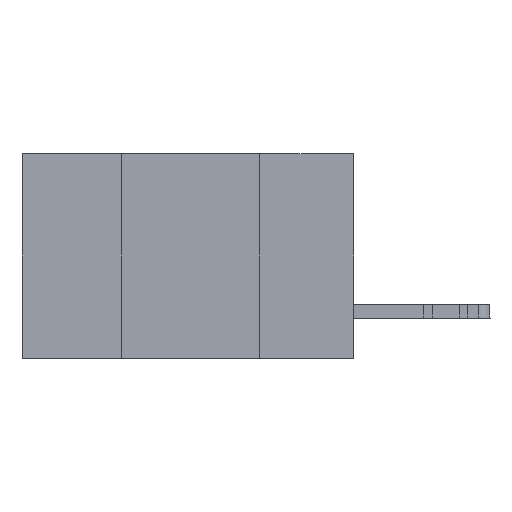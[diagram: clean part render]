
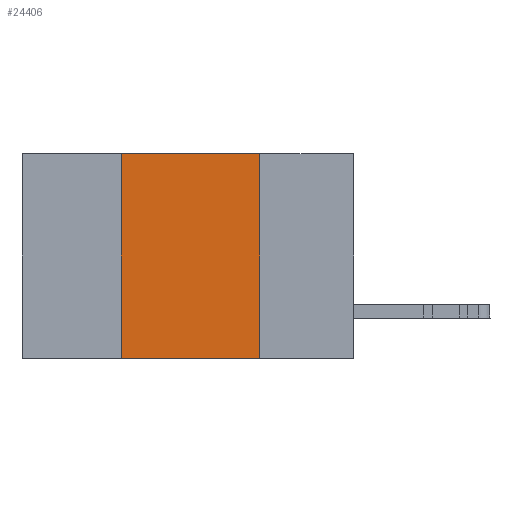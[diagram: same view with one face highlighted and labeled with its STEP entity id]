
A CAD part, left-side view. The second image highlights one B-rep face of the part: STEP entity #24406.
In plain terms, the highlighted planar face has unit normal (-1, 0, 0).
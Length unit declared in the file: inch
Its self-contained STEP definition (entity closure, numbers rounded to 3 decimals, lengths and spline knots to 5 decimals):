
#717 = LINE ( 'NONE', #21312, #35866 ) ;
#966 = EDGE_CURVE ( 'NONE', #1435, #25474, #34516, .T. ) ;
#1435 = VERTEX_POINT ( 'NONE', #48701 ) ;
#3233 = CARTESIAN_POINT ( 'NONE',  ( 0., 0.42, 0. ) ) ;
#5026 = VERTEX_POINT ( 'NONE', #24355 ) ;
#5109 = VECTOR ( 'NONE', #9037, 39.37008 ) ;
#7493 = DIRECTION ( 'NONE',  ( 1., 0., 0. ) ) ;
#9037 = DIRECTION ( 'NONE',  ( 0., -1., 0. ) ) ;
#9723 = AXIS2_PLACEMENT_3D ( 'NONE', #26745, #7493, #50307 ) ;
#10982 = EDGE_CURVE ( 'NONE', #5026, #12121, #717, .T. ) ;
#11799 = ORIENTED_EDGE ( 'NONE', *, *, #35617, .T. ) ;
#12121 = VERTEX_POINT ( 'NONE', #3233 ) ;
#13237 = DIRECTION ( 'NONE',  ( 0., 0., 1. ) ) ;
#15568 = PLANE ( 'NONE',  #9723 ) ;
#20424 = CARTESIAN_POINT ( 'NONE',  ( 0., 0.6, 0. ) ) ;
#20670 = VECTOR ( 'NONE', #24690, 39.37008 ) ;
#21312 = CARTESIAN_POINT ( 'NONE',  ( 0., 0.42, 0. ) ) ;
#24355 = CARTESIAN_POINT ( 'NONE',  ( 0., 0.42, -0.37 ) ) ;
#24406 = ADVANCED_FACE ( 'NONE', ( #31367 ), #15568, .F. ) ;
#24690 = DIRECTION ( 'NONE',  ( 0., -1., 0. ) ) ;
#25474 = VERTEX_POINT ( 'NONE', #46225 ) ;
#26745 = CARTESIAN_POINT ( 'NONE',  ( 0., 0.6, 0. ) ) ;
#30238 = VECTOR ( 'NONE', #38457, 39.37008 ) ;
#30548 = EDGE_LOOP ( 'NONE', ( #31259, #37338, #45623, #11799 ) ) ;
#30609 = CARTESIAN_POINT ( 'NONE',  ( 0., 0.17, 0. ) ) ;
#31259 = ORIENTED_EDGE ( 'NONE', *, *, #966, .F. ) ;
#31367 = FACE_OUTER_BOUND ( 'NONE', #30548, .T. ) ;
#32768 = CARTESIAN_POINT ( 'NONE',  ( 0., 0.6, -0.37 ) ) ;
#34516 = LINE ( 'NONE', #30609, #30238 ) ;
#35278 = EDGE_CURVE ( 'NONE', #12121, #1435, #47140, .T. ) ;
#35617 = EDGE_CURVE ( 'NONE', #5026, #25474, #42716, .T. ) ;
#35866 = VECTOR ( 'NONE', #13237, 39.37008 ) ;
#37338 = ORIENTED_EDGE ( 'NONE', *, *, #35278, .F. ) ;
#38457 = DIRECTION ( 'NONE',  ( 0., 0., -1. ) ) ;
#42716 = LINE ( 'NONE', #32768, #5109 ) ;
#45623 = ORIENTED_EDGE ( 'NONE', *, *, #10982, .F. ) ;
#46225 = CARTESIAN_POINT ( 'NONE',  ( 0., 0.17, -0.37 ) ) ;
#47140 = LINE ( 'NONE', #20424, #20670 ) ;
#48701 = CARTESIAN_POINT ( 'NONE',  ( 0., 0.17, 0. ) ) ;
#50307 = DIRECTION ( 'NONE',  ( 0., 0., -1. ) ) ;
